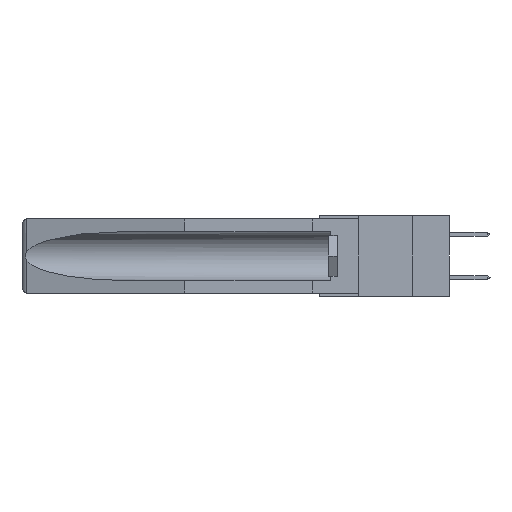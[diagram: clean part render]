
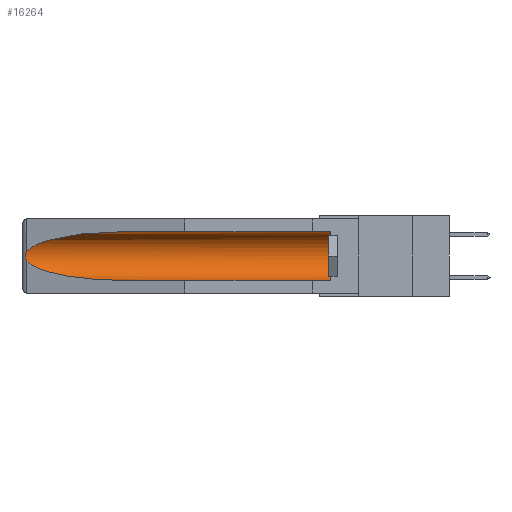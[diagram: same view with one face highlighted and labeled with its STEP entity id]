
A CAD part, left-side view. The second image highlights one B-rep face of the part: STEP entity #16264.
In plain terms, the highlighted cylindrical face has radius 2.857 mm (diameter 5.715 mm), a partial arc.
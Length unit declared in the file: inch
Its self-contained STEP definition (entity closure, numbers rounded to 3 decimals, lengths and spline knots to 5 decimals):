
#555 = CARTESIAN_POINT ( 'NONE',  ( 0.25451, 1.48313, -0.24835 ) ) ;
#669 = FACE_OUTER_BOUND ( 'NONE', #17840, .T. ) ;
#674 = CARTESIAN_POINT ( 'NONE',  ( 0.2673, 1.53269, -0.17917 ) ) ;
#929 = EDGE_CURVE ( 'NONE', #9769, #13687, #14279, .T. ) ;
#1768 = LINE ( 'NONE', #7072, #10401 ) ;
#2220 = CARTESIAN_POINT ( 'NONE',  ( 0.26537, 1.52718, -0.19328 ) ) ;
#2555 = EDGE_CURVE ( 'NONE', #6885, #9769, #7182, .T. ) ;
#2741 = CARTESIAN_POINT ( 'NONE',  ( 0.155, -0.30754, -0.1715 ) ) ;
#3501 = ORIENTED_EDGE ( 'NONE', *, *, #8649, .T. ) ;
#4284 = ORIENTED_EDGE ( 'NONE', *, *, #2555, .T. ) ;
#4555 = EDGE_CURVE ( 'NONE', #11696, #9215, #12160, .T. ) ;
#4708 = ORIENTED_EDGE ( 'NONE', *, *, #4555, .F. ) ;
#5027 = AXIS2_PLACEMENT_3D ( 'NONE', #2741, #5772, #18377 ) ;
#5772 = DIRECTION ( 'NONE',  ( 0., 1., 0. ) ) ;
#6178 = VERTEX_POINT ( 'NONE', #17112 ) ;
#6268 = CARTESIAN_POINT ( 'NONE',  ( 0.26537, 1.52718, -0.14972 ) ) ;
#6720 = CARTESIAN_POINT ( 'NONE',  ( 0.155, 1.07973, -0.059 ) ) ;
#6885 = VERTEX_POINT ( 'NONE', #6720 ) ;
#7072 = CARTESIAN_POINT ( 'NONE',  ( 0.155, -0.30754, -0.059 ) ) ;
#7081 = CARTESIAN_POINT ( 'NONE',  ( 0.2675, 1.53308, -0.16763 ) ) ;
#7182 =( BOUNDED_CURVE ( )  B_SPLINE_CURVE ( 3, ( #17837, #8451, #19482, #12884 ),
 .UNSPECIFIED., .F., .F. ) 
 B_SPLINE_CURVE_WITH_KNOTS ( ( 4, 4 ),
 ( 4.71239, 6.08839 ),
 .UNSPECIFIED. ) 
 CURVE ( )  GEOMETRIC_REPRESENTATION_ITEM ( )  RATIONAL_B_SPLINE_CURVE ( ( 1., 0.848, 0.848, 1. ) ) 
 REPRESENTATION_ITEM ( '' )  );
#7206 = VECTOR ( 'NONE', #7395, 39.37008 ) ;
#7395 = DIRECTION ( 'NONE',  ( 0., 1., 0. ) ) ;
#7828 = CYLINDRICAL_SURFACE ( 'NONE', #5027, 0.1125 ) ;
#7935 = CARTESIAN_POINT ( 'NONE',  ( 0.155, 1.07973, -0.284 ) ) ;
#8406 = DIRECTION ( 'NONE',  ( 0., 0., 1. ) ) ;
#8451 = CARTESIAN_POINT ( 'NONE',  ( 0.21114, 1.30732, -0.059 ) ) ;
#8490 = CARTESIAN_POINT ( 'NONE',  ( 0.155, 1.07973, -0.284 ) ) ;
#8546 = CARTESIAN_POINT ( 'NONE',  ( 0.2675, 1.53308, -0.17534 ) ) ;
#8631 = CARTESIAN_POINT ( 'NONE',  ( 0.26537, 1.52718, -0.19328 ) ) ;
#8649 = EDGE_CURVE ( 'NONE', #13687, #9215, #20325, .T. ) ;
#8920 = CARTESIAN_POINT ( 'NONE',  ( 0.155, -0.30754, -0.284 ) ) ;
#8970 = ORIENTED_EDGE ( 'NONE', *, *, #19364, .T. ) ;
#9215 = VERTEX_POINT ( 'NONE', #7935 ) ;
#9769 = VERTEX_POINT ( 'NONE', #6268 ) ;
#10088 = CARTESIAN_POINT ( 'NONE',  ( 0.26597, 1.52961, -0.15275 ) ) ;
#10102 = CARTESIAN_POINT ( 'NONE',  ( 0.21114, 1.30732, -0.284 ) ) ;
#10198 = DIRECTION ( 'NONE',  ( 0., 1., 0. ) ) ;
#10210 = CARTESIAN_POINT ( 'NONE',  ( 0.26655, 1.53094, -0.18657 ) ) ;
#10401 = VECTOR ( 'NONE', #10198, 39.37008 ) ;
#11502 = EDGE_CURVE ( 'NONE', #6178, #6885, #1768, .T. ) ;
#11696 = VERTEX_POINT ( 'NONE', #14399 ) ;
#12160 = LINE ( 'NONE', #8920, #7206 ) ;
#12446 = CIRCLE ( 'NONE', #13890, 0.1125 ) ;
#12658 = ORIENTED_EDGE ( 'NONE', *, *, #929, .T. ) ;
#12884 = CARTESIAN_POINT ( 'NONE',  ( 0.26537, 1.52718, -0.14972 ) ) ;
#13315 = CARTESIAN_POINT ( 'NONE',  ( 0.26654, 1.53092, -0.15636 ) ) ;
#13423 = CARTESIAN_POINT ( 'NONE',  ( 0.2673, 1.5327, -0.16383 ) ) ;
#13687 = VERTEX_POINT ( 'NONE', #18829 ) ;
#13890 = AXIS2_PLACEMENT_3D ( 'NONE', #17988, #19701, #8406 ) ;
#14279 = B_SPLINE_CURVE_WITH_KNOTS ( 'NONE', 3,
 ( #17992, #10088, #13315, #13423, #7081, #8546, #674, #10210, #18114, #2220 ),
 .UNSPECIFIED., .F., .F.,
 ( 4, 2, 2, 2, 4 ),
 ( 0., 0.00029, 0.00058, 0.00087, 0.00117 ),
 .UNSPECIFIED. ) ;
#14399 = CARTESIAN_POINT ( 'NONE',  ( 0.155, 0.126, -0.284 ) ) ;
#14853 = ORIENTED_EDGE ( 'NONE', *, *, #11502, .T. ) ;
#16264 = ADVANCED_FACE ( 'NONE', ( #669 ), #7828, .F. ) ;
#17112 = CARTESIAN_POINT ( 'NONE',  ( 0.155, 0.126, -0.059 ) ) ;
#17837 = CARTESIAN_POINT ( 'NONE',  ( 0.155, 1.07973, -0.059 ) ) ;
#17840 = EDGE_LOOP ( 'NONE', ( #4284, #12658, #3501, #4708, #8970, #14853 ) ) ;
#17988 = CARTESIAN_POINT ( 'NONE',  ( 0.155, 0.126, -0.1715 ) ) ;
#17992 = CARTESIAN_POINT ( 'NONE',  ( 0.26537, 1.52718, -0.14972 ) ) ;
#18114 = CARTESIAN_POINT ( 'NONE',  ( 0.26597, 1.5296, -0.19026 ) ) ;
#18377 = DIRECTION ( 'NONE',  ( 0., 0., 1. ) ) ;
#18829 = CARTESIAN_POINT ( 'NONE',  ( 0.26537, 1.52718, -0.19328 ) ) ;
#19364 = EDGE_CURVE ( 'NONE', #11696, #6178, #12446, .T. ) ;
#19482 = CARTESIAN_POINT ( 'NONE',  ( 0.25451, 1.48313, -0.09465 ) ) ;
#19701 = DIRECTION ( 'NONE',  ( 0., -1., 0. ) ) ;
#20325 =( BOUNDED_CURVE ( )  B_SPLINE_CURVE ( 3, ( #8631, #555, #10102, #8490 ),
 .UNSPECIFIED., .F., .F. ) 
 B_SPLINE_CURVE_WITH_KNOTS ( ( 4, 4 ),
 ( 0.1948, 1.5708 ),
 .UNSPECIFIED. ) 
 CURVE ( )  GEOMETRIC_REPRESENTATION_ITEM ( )  RATIONAL_B_SPLINE_CURVE ( ( 1., 0.848, 0.848, 1. ) ) 
 REPRESENTATION_ITEM ( '' )  );
